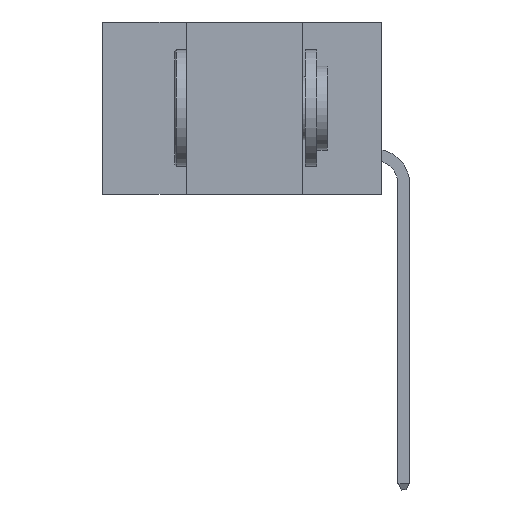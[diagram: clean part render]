
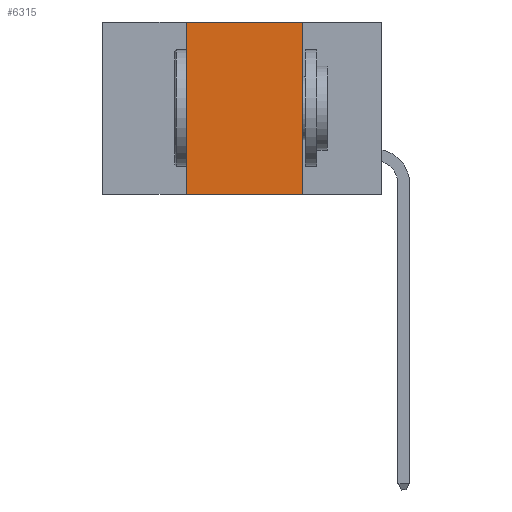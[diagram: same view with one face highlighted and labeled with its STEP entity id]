
A CAD part, left-side view. The second image highlights one B-rep face of the part: STEP entity #6315.
In plain terms, the highlighted planar face has unit normal (-1, 0, 0).
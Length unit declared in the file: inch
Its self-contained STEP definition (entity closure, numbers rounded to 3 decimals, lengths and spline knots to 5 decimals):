
#14 = CARTESIAN_POINT ( 'NONE',  ( 0., 0.17, 0. ) ) ;
#405 = FACE_OUTER_BOUND ( 'NONE', #2736, .T. ) ;
#1551 = DIRECTION ( 'NONE',  ( 0., 0., -1. ) ) ;
#1865 = VERTEX_POINT ( 'NONE', #7279 ) ;
#2127 = VECTOR ( 'NONE', #1551, 39.37008 ) ;
#2457 = CARTESIAN_POINT ( 'NONE',  ( 0., 0.42, 0. ) ) ;
#2547 = EDGE_CURVE ( 'NONE', #9428, #2554, #6702, .T. ) ;
#2554 = VERTEX_POINT ( 'NONE', #10363 ) ;
#2736 = EDGE_LOOP ( 'NONE', ( #5223, #8852, #9536, #9936 ) ) ;
#3725 = CARTESIAN_POINT ( 'NONE',  ( 0., 0.6, 0. ) ) ;
#4094 = EDGE_CURVE ( 'NONE', #7235, #9428, #8787, .T. ) ;
#4591 = VECTOR ( 'NONE', #7005, 39.37008 ) ;
#4624 = DIRECTION ( 'NONE',  ( 0., 0., -1. ) ) ;
#5022 = VECTOR ( 'NONE', #10664, 39.37008 ) ;
#5223 = ORIENTED_EDGE ( 'NONE', *, *, #2547, .F. ) ;
#5261 = CARTESIAN_POINT ( 'NONE',  ( 0., 0.17, 0. ) ) ;
#5870 = DIRECTION ( 'NONE',  ( 0., -1., 0. ) ) ;
#6315 = ADVANCED_FACE ( 'NONE', ( #405 ), #8545, .F. ) ;
#6702 = LINE ( 'NONE', #14, #2127 ) ;
#6790 = VECTOR ( 'NONE', #5870, 39.37008 ) ;
#7005 = DIRECTION ( 'NONE',  ( 0., -1., 0. ) ) ;
#7235 = VERTEX_POINT ( 'NONE', #2457 ) ;
#7254 = LINE ( 'NONE', #10497, #6790 ) ;
#7279 = CARTESIAN_POINT ( 'NONE',  ( 0., 0.42, -0.37 ) ) ;
#7802 = CARTESIAN_POINT ( 'NONE',  ( 0., 0.6, 0. ) ) ;
#8545 = PLANE ( 'NONE',  #9396 ) ;
#8787 = LINE ( 'NONE', #7802, #4591 ) ;
#8798 = EDGE_CURVE ( 'NONE', #1865, #7235, #8935, .T. ) ;
#8852 = ORIENTED_EDGE ( 'NONE', *, *, #4094, .F. ) ;
#8935 = LINE ( 'NONE', #9870, #5022 ) ;
#9326 = DIRECTION ( 'NONE',  ( 1., 0., 0. ) ) ;
#9396 = AXIS2_PLACEMENT_3D ( 'NONE', #3725, #9326, #4624 ) ;
#9428 = VERTEX_POINT ( 'NONE', #5261 ) ;
#9536 = ORIENTED_EDGE ( 'NONE', *, *, #8798, .F. ) ;
#9842 = EDGE_CURVE ( 'NONE', #1865, #2554, #7254, .T. ) ;
#9870 = CARTESIAN_POINT ( 'NONE',  ( 0., 0.42, 0. ) ) ;
#9936 = ORIENTED_EDGE ( 'NONE', *, *, #9842, .T. ) ;
#10363 = CARTESIAN_POINT ( 'NONE',  ( 0., 0.17, -0.37 ) ) ;
#10497 = CARTESIAN_POINT ( 'NONE',  ( 0., 0.6, -0.37 ) ) ;
#10664 = DIRECTION ( 'NONE',  ( 0., 0., 1. ) ) ;
